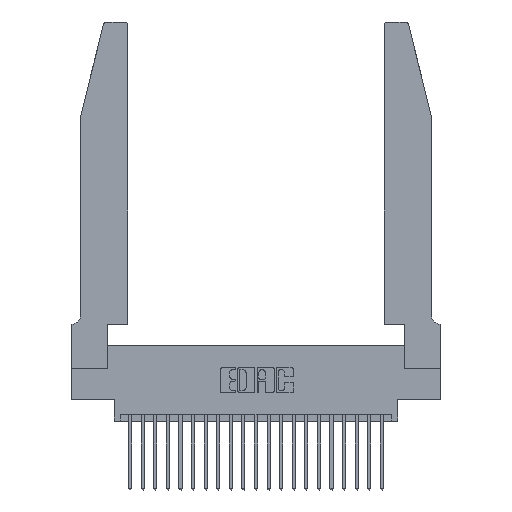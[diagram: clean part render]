
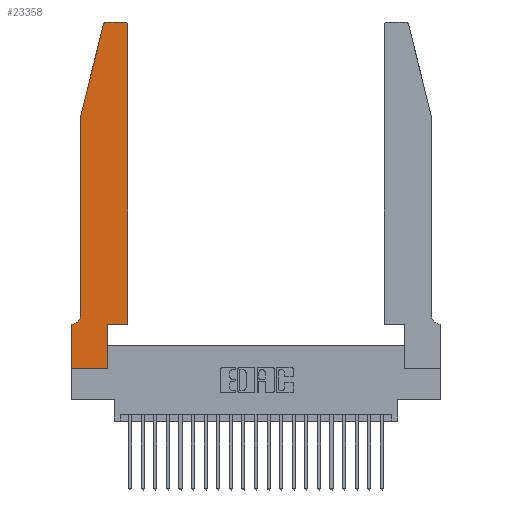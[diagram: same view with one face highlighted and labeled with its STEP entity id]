
A CAD part, top view. The second image highlights one B-rep face of the part: STEP entity #23358.
In plain terms, the highlighted planar face has unit normal (0, 0, 1).
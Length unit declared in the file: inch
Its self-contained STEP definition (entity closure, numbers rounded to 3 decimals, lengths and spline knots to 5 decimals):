
#261 = DIRECTION ( 'NONE',  ( 1., 0., 0. ) ) ;
#366 = ORIENTED_EDGE ( 'NONE', *, *, #16083, .T. ) ;
#382 = CARTESIAN_POINT ( 'NONE',  ( 0.25487, 2.72718, 0.37 ) ) ;
#403 = DIRECTION ( 'NONE',  ( 1., 0., 0. ) ) ;
#652 = DIRECTION ( 'NONE',  ( 0., 1., 0. ) ) ;
#661 = VECTOR ( 'NONE', #7559, 39.37008 ) ;
#681 = DIRECTION ( 'NONE',  ( -1., 0., 0. ) ) ;
#1193 = ORIENTED_EDGE ( 'NONE', *, *, #16307, .T. ) ;
#1871 = AXIS2_PLACEMENT_3D ( 'NONE', #21678, #8719, #21838 ) ;
#1983 = VECTOR ( 'NONE', #3244, 39.37008 ) ;
#2465 = CARTESIAN_POINT ( 'NONE',  ( 0.0055, 0.42, 0.37 ) ) ;
#2471 = DIRECTION ( 'NONE',  ( 0., -1., 0. ) ) ;
#2495 = VERTEX_POINT ( 'NONE', #11016 ) ;
#2498 = EDGE_CURVE ( 'NONE', #16982, #3424, #22924, .T. ) ;
#2813 = VERTEX_POINT ( 'NONE', #16174 ) ;
#2909 = ORIENTED_EDGE ( 'NONE', *, *, #13476, .T. ) ;
#3244 = DIRECTION ( 'NONE',  ( 0., 1., 0. ) ) ;
#3309 = EDGE_CURVE ( 'NONE', #19778, #2495, #8497, .T. ) ;
#3424 = VERTEX_POINT ( 'NONE', #14583 ) ;
#4099 = LINE ( 'NONE', #10295, #23476 ) ;
#4433 = ORIENTED_EDGE ( 'NONE', *, *, #9378, .T. ) ;
#4474 = EDGE_CURVE ( 'NONE', #14662, #2813, #15195, .T. ) ;
#4486 = CIRCLE ( 'NONE', #19674, 0.07 ) ;
#4865 = ORIENTED_EDGE ( 'NONE', *, *, #17616, .T. ) ;
#5226 = AXIS2_PLACEMENT_3D ( 'NONE', #11457, #21100, #9816 ) ;
#5576 = CARTESIAN_POINT ( 'NONE',  ( 0., 0., 0.37 ) ) ;
#5700 = EDGE_CURVE ( 'NONE', #2495, #11906, #14872, .T. ) ;
#5953 = LINE ( 'NONE', #6072, #20332 ) ;
#6072 = CARTESIAN_POINT ( 'NONE',  ( 0., 0., 0.37 ) ) ;
#6690 = AXIS2_PLACEMENT_3D ( 'NONE', #22822, #18898, #403 ) ;
#7464 = ORIENTED_EDGE ( 'NONE', *, *, #3309, .T. ) ;
#7559 = DIRECTION ( 'NONE',  ( 0., -1., 0. ) ) ;
#7582 = EDGE_LOOP ( 'NONE', ( #4433, #4865, #7464, #9382, #2909, #366, #13298, #21422, #15849, #19134, #10119, #1193 ) ) ;
#7911 = VECTOR ( 'NONE', #8956, 39.37008 ) ;
#8439 = VERTEX_POINT ( 'NONE', #8504 ) ;
#8497 = LINE ( 'NONE', #10777, #7911 ) ;
#8504 = CARTESIAN_POINT ( 'NONE',  ( 0.4505, 0.35, 0.37 ) ) ;
#8719 = DIRECTION ( 'NONE',  ( 0., 0., 1. ) ) ;
#8956 = DIRECTION ( 'NONE',  ( -0.239, -0.971, 0. ) ) ;
#9055 = EDGE_CURVE ( 'NONE', #8439, #10224, #4099, .T. ) ;
#9228 = VECTOR ( 'NONE', #2471, 39.37008 ) ;
#9378 = EDGE_CURVE ( 'NONE', #22177, #19839, #22006, .T. ) ;
#9382 = ORIENTED_EDGE ( 'NONE', *, *, #5700, .T. ) ;
#9778 = DIRECTION ( 'NONE',  ( 1., 0., 0. ) ) ;
#9816 = DIRECTION ( 'NONE',  ( 1., 0., 0. ) ) ;
#10119 = ORIENTED_EDGE ( 'NONE', *, *, #9055, .T. ) ;
#10224 = VERTEX_POINT ( 'NONE', #15827 ) ;
#10295 = CARTESIAN_POINT ( 'NONE',  ( 0.4505, 0.35, 0.37 ) ) ;
#10777 = CARTESIAN_POINT ( 'NONE',  ( 0.0755, 2., 0.37 ) ) ;
#11016 = CARTESIAN_POINT ( 'NONE',  ( 0.0755, 2., 0.37 ) ) ;
#11457 = CARTESIAN_POINT ( 'NONE',  ( 0., 0.35, 0.37 ) ) ;
#11672 = CARTESIAN_POINT ( 'NONE',  ( 0.284, 2.75, 0.37 ) ) ;
#11906 = VERTEX_POINT ( 'NONE', #19081 ) ;
#11963 = FACE_OUTER_BOUND ( 'NONE', #7582, .T. ) ;
#11972 = DIRECTION ( 'NONE',  ( 0., 0., -1. ) ) ;
#12326 = LINE ( 'NONE', #23788, #17898 ) ;
#12610 = DIRECTION ( 'NONE',  ( -1., 0., 0. ) ) ;
#12664 = DIRECTION ( 'NONE',  ( -1., 0., 0. ) ) ;
#12720 = EDGE_CURVE ( 'NONE', #3424, #14662, #5953, .T. ) ;
#13298 = ORIENTED_EDGE ( 'NONE', *, *, #2498, .T. ) ;
#13366 = CARTESIAN_POINT ( 'NONE',  ( 0.4505, 0.35, 0.37 ) ) ;
#13476 = EDGE_CURVE ( 'NONE', #11906, #20206, #4486, .T. ) ;
#13962 = CARTESIAN_POINT ( 'NONE',  ( 0.0755, 2., 0.37 ) ) ;
#14517 = CARTESIAN_POINT ( 'NONE',  ( 0.2865, 0.35, 0.37 ) ) ;
#14583 = CARTESIAN_POINT ( 'NONE',  ( 0., 0., 0.37 ) ) ;
#14662 = VERTEX_POINT ( 'NONE', #14965 ) ;
#14755 = EDGE_CURVE ( 'NONE', #2813, #8439, #20872, .T. ) ;
#14872 = LINE ( 'NONE', #13962, #9228 ) ;
#14965 = CARTESIAN_POINT ( 'NONE',  ( 0.2865, 0., 0.37 ) ) ;
#15195 = LINE ( 'NONE', #14517, #1983 ) ;
#15827 = CARTESIAN_POINT ( 'NONE',  ( 0.4505, 2.72, 0.37 ) ) ;
#15849 = ORIENTED_EDGE ( 'NONE', *, *, #4474, .T. ) ;
#15919 = VECTOR ( 'NONE', #261, 39.37008 ) ;
#16083 = EDGE_CURVE ( 'NONE', #20206, #16982, #12326, .T. ) ;
#16174 = CARTESIAN_POINT ( 'NONE',  ( 0.2865, 0.35, 0.37 ) ) ;
#16307 = EDGE_CURVE ( 'NONE', #10224, #22177, #19920, .T. ) ;
#16982 = VERTEX_POINT ( 'NONE', #20205 ) ;
#17014 = VECTOR ( 'NONE', #12664, 39.37008 ) ;
#17375 = CARTESIAN_POINT ( 'NONE',  ( 0.0055, 0.35, 0.37 ) ) ;
#17616 = EDGE_CURVE ( 'NONE', #19839, #19778, #18650, .T. ) ;
#17898 = VECTOR ( 'NONE', #12610, 39.37008 ) ;
#18650 = CIRCLE ( 'NONE', #1871, 0.03 ) ;
#18898 = DIRECTION ( 'NONE',  ( 0., 0., 1. ) ) ;
#19081 = CARTESIAN_POINT ( 'NONE',  ( 0.0755, 0.42, 0.37 ) ) ;
#19134 = ORIENTED_EDGE ( 'NONE', *, *, #14755, .T. ) ;
#19674 = AXIS2_PLACEMENT_3D ( 'NONE', #2465, #11972, #681 ) ;
#19778 = VERTEX_POINT ( 'NONE', #382 ) ;
#19839 = VERTEX_POINT ( 'NONE', #11672 ) ;
#19920 = CIRCLE ( 'NONE', #6690, 0.03 ) ;
#20205 = CARTESIAN_POINT ( 'NONE',  ( 0., 0.35, 0.37 ) ) ;
#20206 = VERTEX_POINT ( 'NONE', #17375 ) ;
#20332 = VECTOR ( 'NONE', #9778, 39.37008 ) ;
#20486 = CARTESIAN_POINT ( 'NONE',  ( 0.4205, 2.75, 0.37 ) ) ;
#20872 = LINE ( 'NONE', #13366, #15919 ) ;
#20931 = PLANE ( 'NONE',  #5226 ) ;
#21100 = DIRECTION ( 'NONE',  ( 0., 0., 1. ) ) ;
#21422 = ORIENTED_EDGE ( 'NONE', *, *, #12720, .T. ) ;
#21678 = CARTESIAN_POINT ( 'NONE',  ( 0.284, 2.72, 0.37 ) ) ;
#21838 = DIRECTION ( 'NONE',  ( 1., 0., 0. ) ) ;
#22006 = LINE ( 'NONE', #22145, #17014 ) ;
#22145 = CARTESIAN_POINT ( 'NONE',  ( 0.2605, 2.75, 0.37 ) ) ;
#22177 = VERTEX_POINT ( 'NONE', #20486 ) ;
#22822 = CARTESIAN_POINT ( 'NONE',  ( 0.4205, 2.72, 0.37 ) ) ;
#22924 = LINE ( 'NONE', #5576, #661 ) ;
#23358 = ADVANCED_FACE ( 'NONE', ( #11963 ), #20931, .T. ) ;
#23476 = VECTOR ( 'NONE', #652, 39.37008 ) ;
#23788 = CARTESIAN_POINT ( 'NONE',  ( 0.0755, 0.35, 0.37 ) ) ;
